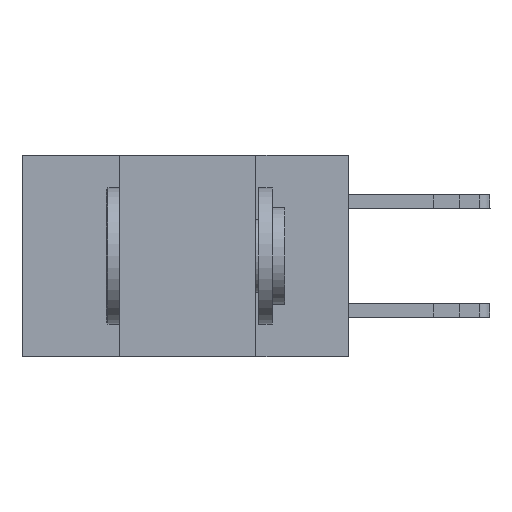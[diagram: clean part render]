
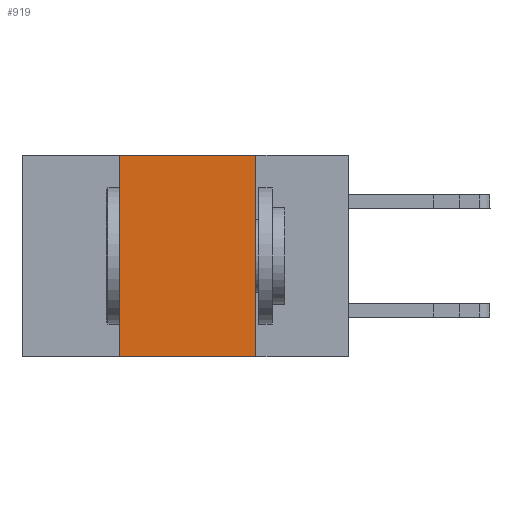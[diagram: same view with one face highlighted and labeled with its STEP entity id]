
A CAD part, left-side view. The second image highlights one B-rep face of the part: STEP entity #919.
In plain terms, the highlighted planar face has unit normal (-1, 0, 0).
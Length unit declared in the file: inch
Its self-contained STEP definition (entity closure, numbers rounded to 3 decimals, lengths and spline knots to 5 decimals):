
#146 = ORIENTED_EDGE ( 'NONE', *, *, #6102, .T. ) ;
#324 = PLANE ( 'NONE',  #6363 ) ;
#919 = ADVANCED_FACE ( 'NONE', ( #9268 ), #324, .F. ) ;
#1541 = VECTOR ( 'NONE', #4453, 39.37008 ) ;
#1609 = CARTESIAN_POINT ( 'NONE',  ( 0., 0.42, -0.37 ) ) ;
#1820 = LINE ( 'NONE', #11606, #6280 ) ;
#1906 = CARTESIAN_POINT ( 'NONE',  ( 0., 0.17, -0.37 ) ) ;
#2741 = CARTESIAN_POINT ( 'NONE',  ( 0., 0.42, 0. ) ) ;
#3262 = DIRECTION ( 'NONE',  ( 1., 0., 0. ) ) ;
#3340 = VECTOR ( 'NONE', #10826, 39.37008 ) ;
#3348 = EDGE_LOOP ( 'NONE', ( #4288, #7904, #12341, #146 ) ) ;
#3563 = LINE ( 'NONE', #8450, #8952 ) ;
#3625 = VERTEX_POINT ( 'NONE', #7458 ) ;
#3647 = EDGE_CURVE ( 'NONE', #11607, #3625, #3563, .T. ) ;
#4170 = EDGE_CURVE ( 'NONE', #3625, #10060, #4678, .T. ) ;
#4232 = CARTESIAN_POINT ( 'NONE',  ( 0., 0.6, 0. ) ) ;
#4288 = ORIENTED_EDGE ( 'NONE', *, *, #4170, .F. ) ;
#4453 = DIRECTION ( 'NONE',  ( 0., 0., 1. ) ) ;
#4678 = LINE ( 'NONE', #6724, #3340 ) ;
#4985 = EDGE_CURVE ( 'NONE', #6484, #11607, #5429, .T. ) ;
#5388 = DIRECTION ( 'NONE',  ( 0., 0., -1. ) ) ;
#5429 = LINE ( 'NONE', #9436, #1541 ) ;
#6102 = EDGE_CURVE ( 'NONE', #6484, #10060, #1820, .T. ) ;
#6280 = VECTOR ( 'NONE', #6666, 39.37008 ) ;
#6363 = AXIS2_PLACEMENT_3D ( 'NONE', #4232, #3262, #5388 ) ;
#6484 = VERTEX_POINT ( 'NONE', #1609 ) ;
#6666 = DIRECTION ( 'NONE',  ( 0., -1., 0. ) ) ;
#6724 = CARTESIAN_POINT ( 'NONE',  ( 0., 0.17, -0.37 ) ) ;
#7458 = CARTESIAN_POINT ( 'NONE',  ( 0., 0.17, 0. ) ) ;
#7904 = ORIENTED_EDGE ( 'NONE', *, *, #3647, .F. ) ;
#8450 = CARTESIAN_POINT ( 'NONE',  ( 0., 0.6, 0. ) ) ;
#8952 = VECTOR ( 'NONE', #10537, 39.37008 ) ;
#9268 = FACE_OUTER_BOUND ( 'NONE', #3348, .T. ) ;
#9436 = CARTESIAN_POINT ( 'NONE',  ( 0., 0.42, -0.37 ) ) ;
#10060 = VERTEX_POINT ( 'NONE', #1906 ) ;
#10537 = DIRECTION ( 'NONE',  ( 0., -1., 0. ) ) ;
#10826 = DIRECTION ( 'NONE',  ( 0., 0., -1. ) ) ;
#11606 = CARTESIAN_POINT ( 'NONE',  ( 0., 0.6, -0.37 ) ) ;
#11607 = VERTEX_POINT ( 'NONE', #2741 ) ;
#12341 = ORIENTED_EDGE ( 'NONE', *, *, #4985, .F. ) ;
